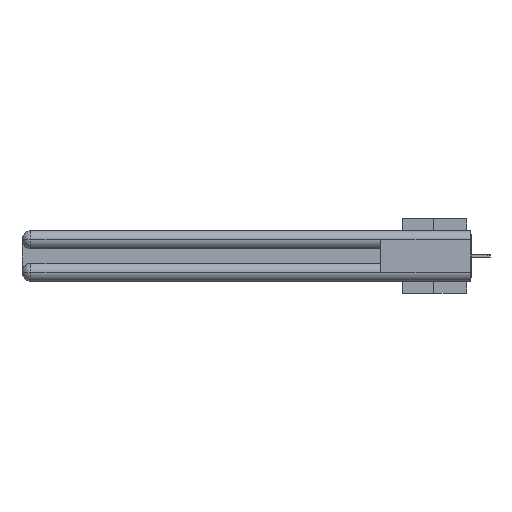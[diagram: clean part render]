
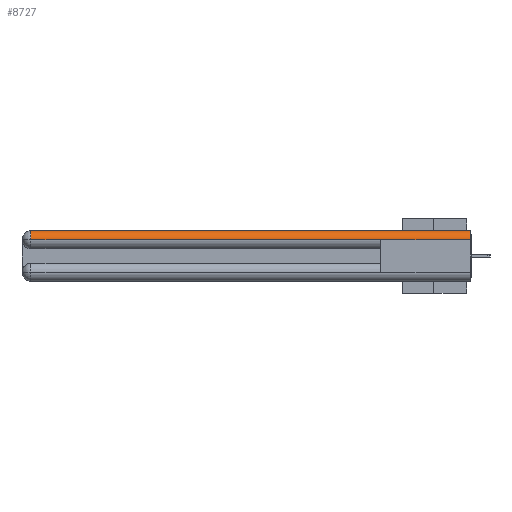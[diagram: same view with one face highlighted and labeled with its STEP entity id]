
A CAD part, left-side view. The second image highlights one B-rep face of the part: STEP entity #8727.
In plain terms, the highlighted cylindrical face has radius 1.562 mm (diameter 3.124 mm), a partial arc.
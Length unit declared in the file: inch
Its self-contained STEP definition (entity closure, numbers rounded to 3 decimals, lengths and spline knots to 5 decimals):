
#73 = DIRECTION ( 'NONE',  ( 0., -1., 0. ) ) ;
#813 = CARTESIAN_POINT ( 'NONE',  ( 0., 0.6, -0.0615 ) ) ;
#1446 = DIRECTION ( 'NONE',  ( 0., -1., 0. ) ) ;
#2078 = VERTEX_POINT ( 'NONE', #813 ) ;
#2236 = DIRECTION ( 'NONE',  ( 1., 0., 0. ) ) ;
#2987 = VERTEX_POINT ( 'NONE', #4609 ) ;
#4376 = LINE ( 'NONE', #6322, #18762 ) ;
#4609 = CARTESIAN_POINT ( 'NONE',  ( 0.0615, 0., 0. ) ) ;
#5390 = ORIENTED_EDGE ( 'NONE', *, *, #6879, .T. ) ;
#5672 = DIRECTION ( 'NONE',  ( 0., 1., 0. ) ) ;
#6322 = CARTESIAN_POINT ( 'NONE',  ( 0., 3., -0.0615 ) ) ;
#6879 = EDGE_CURVE ( 'NONE', #13432, #2078, #4376, .T. ) ;
#7041 = EDGE_CURVE ( 'NONE', #21446, #2078, #35063, .T. ) ;
#7698 = LINE ( 'NONE', #34279, #21107 ) ;
#8727 = ADVANCED_FACE ( 'NONE', ( #15108 ), #21706, .T. ) ;
#9946 = AXIS2_PLACEMENT_3D ( 'NONE', #18701, #1446, #21540 ) ;
#10805 = EDGE_CURVE ( 'NONE', #34129, #2987, #7698, .T. ) ;
#11731 = EDGE_CURVE ( 'NONE', #34129, #13432, #36474, .T. ) ;
#12252 = ORIENTED_EDGE ( 'NONE', *, *, #11731, .T. ) ;
#12563 = VECTOR ( 'NONE', #29704, 39.37008 ) ;
#12826 = CARTESIAN_POINT ( 'NONE',  ( 0., 3., -0.0615 ) ) ;
#13432 = VERTEX_POINT ( 'NONE', #14777 ) ;
#13647 = CARTESIAN_POINT ( 'NONE',  ( 0.0615, 2.94, 0. ) ) ;
#14777 = CARTESIAN_POINT ( 'NONE',  ( 0., 2.94, -0.0615 ) ) ;
#14947 = ORIENTED_EDGE ( 'NONE', *, *, #30808, .F. ) ;
#15108 = FACE_OUTER_BOUND ( 'NONE', #18320, .T. ) ;
#18302 = CARTESIAN_POINT ( 'NONE',  ( 0., 0., -0.0615 ) ) ;
#18320 = EDGE_LOOP ( 'NONE', ( #18890, #12252, #5390, #29030, #14947 ) ) ;
#18701 = CARTESIAN_POINT ( 'NONE',  ( 0.0615, 2.94, -0.0615 ) ) ;
#18762 = VECTOR ( 'NONE', #31802, 39.37008 ) ;
#18890 = ORIENTED_EDGE ( 'NONE', *, *, #10805, .F. ) ;
#18946 = AXIS2_PLACEMENT_3D ( 'NONE', #36944, #5672, #31297 ) ;
#19462 = DIRECTION ( 'NONE',  ( 0., -1., 0. ) ) ;
#20307 = AXIS2_PLACEMENT_3D ( 'NONE', #36328, #19462, #2236 ) ;
#21107 = VECTOR ( 'NONE', #73, 39.37008 ) ;
#21240 = CIRCLE ( 'NONE', #20307, 0.0615 ) ;
#21446 = VERTEX_POINT ( 'NONE', #18302 ) ;
#21540 = DIRECTION ( 'NONE',  ( 0., 0., 1. ) ) ;
#21706 = CYLINDRICAL_SURFACE ( 'NONE', #18946, 0.0615 ) ;
#29030 = ORIENTED_EDGE ( 'NONE', *, *, #7041, .F. ) ;
#29704 = DIRECTION ( 'NONE',  ( 0., 1., 0. ) ) ;
#30808 = EDGE_CURVE ( 'NONE', #2987, #21446, #21240, .T. ) ;
#31297 = DIRECTION ( 'NONE',  ( 0., 0., 1. ) ) ;
#31802 = DIRECTION ( 'NONE',  ( 0., -1., 0. ) ) ;
#34129 = VERTEX_POINT ( 'NONE', #13647 ) ;
#34279 = CARTESIAN_POINT ( 'NONE',  ( 0.0615, 0., 0. ) ) ;
#35063 = LINE ( 'NONE', #12826, #12563 ) ;
#36328 = CARTESIAN_POINT ( 'NONE',  ( 0.0615, 0., -0.0615 ) ) ;
#36474 = CIRCLE ( 'NONE', #9946, 0.0615 ) ;
#36944 = CARTESIAN_POINT ( 'NONE',  ( 0.0615, 0., -0.0615 ) ) ;
